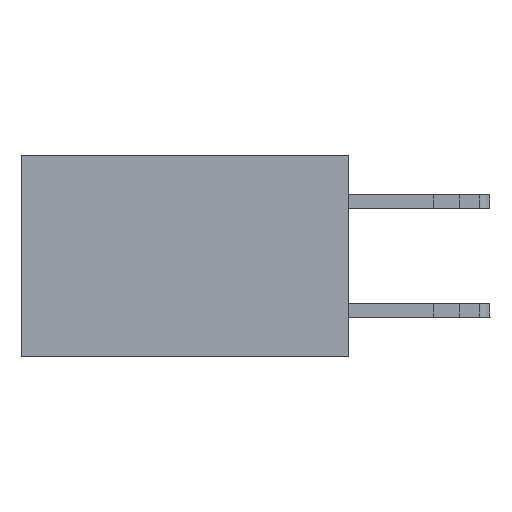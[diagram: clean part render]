
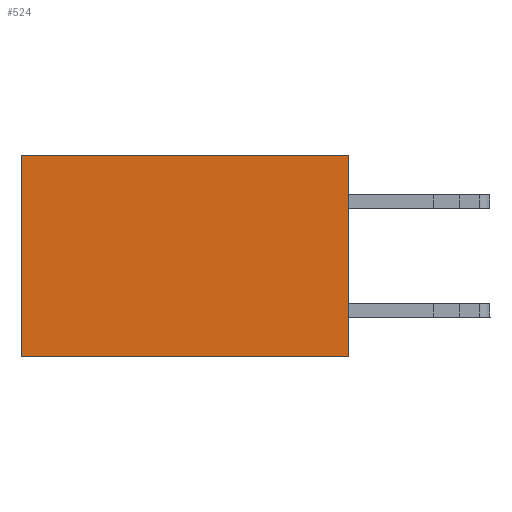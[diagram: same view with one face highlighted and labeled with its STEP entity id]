
A CAD part, left-side view. The second image highlights one B-rep face of the part: STEP entity #524.
In plain terms, the highlighted planar face has unit normal (-1, 0, 0).
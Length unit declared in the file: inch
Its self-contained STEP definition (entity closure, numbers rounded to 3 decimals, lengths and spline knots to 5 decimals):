
#524 = ADVANCED_FACE ( 'NONE', ( #16705 ), #12030, .F. ) ;
#920 = DIRECTION ( 'NONE',  ( 0., 1., 0. ) ) ;
#1387 = AXIS2_PLACEMENT_3D ( 'NONE', #8493, #10344, #1492 ) ;
#1492 = DIRECTION ( 'NONE',  ( 0., 0., -1. ) ) ;
#1608 = DIRECTION ( 'NONE',  ( 0., 0., -1. ) ) ;
#2093 = VECTOR ( 'NONE', #22219, 39.37008 ) ;
#4123 = VERTEX_POINT ( 'NONE', #9521 ) ;
#4464 = LINE ( 'NONE', #20735, #17825 ) ;
#6094 = ORIENTED_EDGE ( 'NONE', *, *, #10617, .F. ) ;
#6615 = CARTESIAN_POINT ( 'NONE',  ( 0.298, 0.6, 0. ) ) ;
#6856 = LINE ( 'NONE', #10743, #19692 ) ;
#8493 = CARTESIAN_POINT ( 'NONE',  ( 0.298, 0., 0. ) ) ;
#8774 = EDGE_CURVE ( 'NONE', #4123, #14320, #11385, .T. ) ;
#8807 = VERTEX_POINT ( 'NONE', #11891 ) ;
#9521 = CARTESIAN_POINT ( 'NONE',  ( 0.298, 0.6, 0. ) ) ;
#10344 = DIRECTION ( 'NONE',  ( 1., 0., 0. ) ) ;
#10617 = EDGE_CURVE ( 'NONE', #21254, #8807, #4464, .T. ) ;
#10743 = CARTESIAN_POINT ( 'NONE',  ( 0.298, 0., -0.37 ) ) ;
#11003 = CARTESIAN_POINT ( 'NONE',  ( 0.298, 0.6, -0.37 ) ) ;
#11035 = ORIENTED_EDGE ( 'NONE', *, *, #8774, .T. ) ;
#11385 = LINE ( 'NONE', #6615, #2093 ) ;
#11891 = CARTESIAN_POINT ( 'NONE',  ( 0.298, 0., -0.37 ) ) ;
#12030 = PLANE ( 'NONE',  #1387 ) ;
#12192 = EDGE_CURVE ( 'NONE', #8807, #14320, #6856, .T. ) ;
#12494 = DIRECTION ( 'NONE',  ( 0., 1., 0. ) ) ;
#13225 = EDGE_CURVE ( 'NONE', #21254, #4123, #22078, .T. ) ;
#14320 = VERTEX_POINT ( 'NONE', #11003 ) ;
#15012 = VECTOR ( 'NONE', #920, 39.37008 ) ;
#16705 = FACE_OUTER_BOUND ( 'NONE', #17046, .T. ) ;
#17046 = EDGE_LOOP ( 'NONE', ( #11035, #21358, #6094, #17580 ) ) ;
#17580 = ORIENTED_EDGE ( 'NONE', *, *, #13225, .T. ) ;
#17825 = VECTOR ( 'NONE', #1608, 39.37008 ) ;
#18347 = CARTESIAN_POINT ( 'NONE',  ( 0.298, 0., 0. ) ) ;
#19692 = VECTOR ( 'NONE', #12494, 39.37008 ) ;
#20139 = CARTESIAN_POINT ( 'NONE',  ( 0.298, 0., 0. ) ) ;
#20735 = CARTESIAN_POINT ( 'NONE',  ( 0.298, 0., 0. ) ) ;
#21254 = VERTEX_POINT ( 'NONE', #18347 ) ;
#21358 = ORIENTED_EDGE ( 'NONE', *, *, #12192, .F. ) ;
#22078 = LINE ( 'NONE', #20139, #15012 ) ;
#22219 = DIRECTION ( 'NONE',  ( 0., 0., -1. ) ) ;
